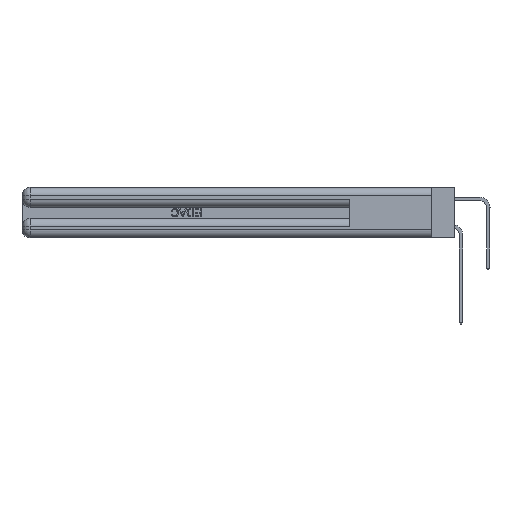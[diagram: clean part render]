
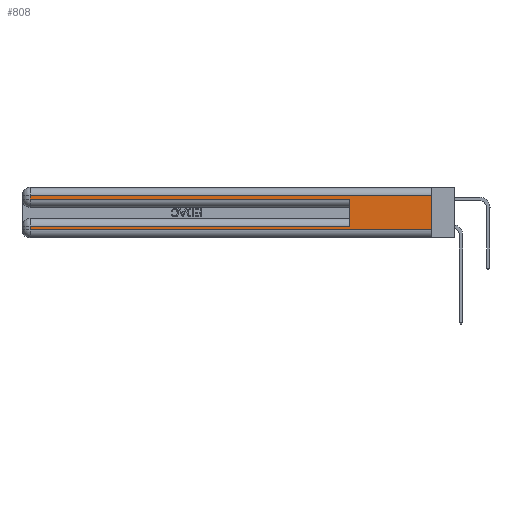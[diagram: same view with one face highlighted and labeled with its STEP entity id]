
A CAD part, left-side view. The second image highlights one B-rep face of the part: STEP entity #808.
In plain terms, the highlighted planar face has unit normal (-1, 0, 0).
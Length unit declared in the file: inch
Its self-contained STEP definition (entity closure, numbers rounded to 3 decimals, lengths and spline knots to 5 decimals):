
#419 = DIRECTION ( 'NONE',  ( 0., 0., -1. ) ) ;
#563 = ORIENTED_EDGE ( 'NONE', *, *, #686, .T. ) ;
#686 = EDGE_CURVE ( 'NONE', #25862, #13405, #5065, .T. ) ;
#808 = ADVANCED_FACE ( 'NONE', ( #45400 ), #28209, .F. ) ;
#1660 = LINE ( 'NONE', #13838, #38038 ) ;
#3790 = LINE ( 'NONE', #35758, #29159 ) ;
#4180 = VERTEX_POINT ( 'NONE', #32944 ) ;
#5065 = LINE ( 'NONE', #11934, #11373 ) ;
#5760 = AXIS2_PLACEMENT_3D ( 'NONE', #20782, #35312, #28048 ) ;
#9397 = CARTESIAN_POINT ( 'NONE',  ( 0., 0., 0.285 ) ) ;
#10394 = VERTEX_POINT ( 'NONE', #24185 ) ;
#10496 = CARTESIAN_POINT ( 'NONE',  ( 0., 2.94, 0.06 ) ) ;
#11373 = VECTOR ( 'NONE', #40789, 39.37008 ) ;
#11582 = EDGE_CURVE ( 'NONE', #37370, #13405, #16744, .T. ) ;
#11934 = CARTESIAN_POINT ( 'NONE',  ( 0., 0., 0.06 ) ) ;
#12991 = DIRECTION ( 'NONE',  ( 0., -1., 0. ) ) ;
#13405 = VERTEX_POINT ( 'NONE', #25256 ) ;
#13660 = DIRECTION ( 'NONE',  ( 0., 0., -1. ) ) ;
#13838 = CARTESIAN_POINT ( 'NONE',  ( 0., 0., 0.31 ) ) ;
#14026 = ORIENTED_EDGE ( 'NONE', *, *, #24065, .F. ) ;
#14815 = ORIENTED_EDGE ( 'NONE', *, *, #33475, .T. ) ;
#15908 = ORIENTED_EDGE ( 'NONE', *, *, #28259, .T. ) ;
#16488 = LINE ( 'NONE', #9397, #28595 ) ;
#16744 = LINE ( 'NONE', #22508, #31179 ) ;
#16875 = VERTEX_POINT ( 'NONE', #29741 ) ;
#18295 = LINE ( 'NONE', #41850, #33287 ) ;
#19745 = DIRECTION ( 'NONE',  ( 0., 1., 0. ) ) ;
#20782 = CARTESIAN_POINT ( 'NONE',  ( 0., 0., 0.37 ) ) ;
#20885 = DIRECTION ( 'NONE',  ( 0., 0., -1. ) ) ;
#22508 = CARTESIAN_POINT ( 'NONE',  ( 0., 0., 0.37 ) ) ;
#22740 = EDGE_CURVE ( 'NONE', #4180, #26139, #41285, .T. ) ;
#22961 = EDGE_CURVE ( 'NONE', #10394, #25862, #3790, .T. ) ;
#24065 = EDGE_CURVE ( 'NONE', #36677, #16875, #27961, .T. ) ;
#24185 = CARTESIAN_POINT ( 'NONE',  ( 0., 2.94, 0.085 ) ) ;
#24382 = ORIENTED_EDGE ( 'NONE', *, *, #22740, .T. ) ;
#25256 = CARTESIAN_POINT ( 'NONE',  ( 0., 0., 0.06 ) ) ;
#25862 = VERTEX_POINT ( 'NONE', #10496 ) ;
#26139 = VERTEX_POINT ( 'NONE', #33896 ) ;
#26839 = ORIENTED_EDGE ( 'NONE', *, *, #47421, .T. ) ;
#27961 = LINE ( 'NONE', #43393, #46924 ) ;
#28048 = DIRECTION ( 'NONE',  ( 0., 0., -1. ) ) ;
#28209 = PLANE ( 'NONE',  #5760 ) ;
#28259 = EDGE_CURVE ( 'NONE', #36677, #10394, #18295, .T. ) ;
#28595 = VECTOR ( 'NONE', #12991, 39.37008 ) ;
#29059 = DIRECTION ( 'NONE',  ( 0., 0., 1. ) ) ;
#29159 = VECTOR ( 'NONE', #13660, 39.37008 ) ;
#29741 = CARTESIAN_POINT ( 'NONE',  ( 0., 0.6, 0.285 ) ) ;
#30626 = EDGE_LOOP ( 'NONE', ( #44843, #14815, #24382, #26839, #14026, #15908, #41473, #563 ) ) ;
#31179 = VECTOR ( 'NONE', #419, 39.37008 ) ;
#31740 = CARTESIAN_POINT ( 'NONE',  ( 0., 2.94, 0.37 ) ) ;
#32944 = CARTESIAN_POINT ( 'NONE',  ( 0., 2.94, 0.31 ) ) ;
#33287 = VECTOR ( 'NONE', #19745, 39.37008 ) ;
#33475 = EDGE_CURVE ( 'NONE', #37370, #4180, #1660, .T. ) ;
#33896 = CARTESIAN_POINT ( 'NONE',  ( 0., 2.94, 0.285 ) ) ;
#35312 = DIRECTION ( 'NONE',  ( 1., 0., 0. ) ) ;
#35457 = DIRECTION ( 'NONE',  ( 0., 1., 0. ) ) ;
#35758 = CARTESIAN_POINT ( 'NONE',  ( 0., 2.94, 0.37 ) ) ;
#36111 = VECTOR ( 'NONE', #20885, 39.37008 ) ;
#36677 = VERTEX_POINT ( 'NONE', #42971 ) ;
#37370 = VERTEX_POINT ( 'NONE', #47557 ) ;
#38038 = VECTOR ( 'NONE', #35457, 39.37008 ) ;
#40789 = DIRECTION ( 'NONE',  ( 0., -1., 0. ) ) ;
#41285 = LINE ( 'NONE', #31740, #36111 ) ;
#41473 = ORIENTED_EDGE ( 'NONE', *, *, #22961, .T. ) ;
#41850 = CARTESIAN_POINT ( 'NONE',  ( 0., 0., 0.085 ) ) ;
#42971 = CARTESIAN_POINT ( 'NONE',  ( 0., 0.6, 0.085 ) ) ;
#43393 = CARTESIAN_POINT ( 'NONE',  ( 0., 0.6, 0.145 ) ) ;
#44843 = ORIENTED_EDGE ( 'NONE', *, *, #11582, .F. ) ;
#45400 = FACE_OUTER_BOUND ( 'NONE', #30626, .T. ) ;
#46924 = VECTOR ( 'NONE', #29059, 39.37008 ) ;
#47421 = EDGE_CURVE ( 'NONE', #26139, #16875, #16488, .T. ) ;
#47557 = CARTESIAN_POINT ( 'NONE',  ( 0., 0., 0.31 ) ) ;
